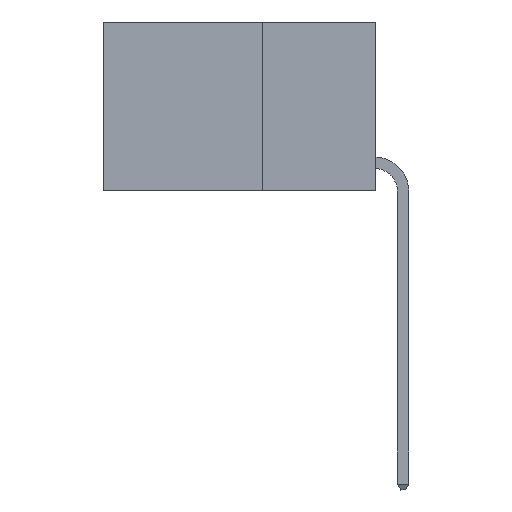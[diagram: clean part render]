
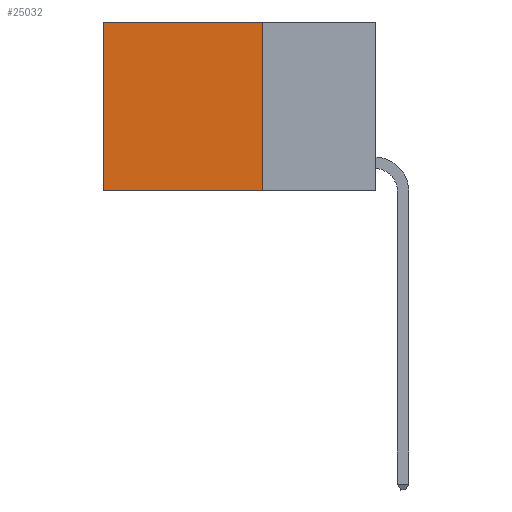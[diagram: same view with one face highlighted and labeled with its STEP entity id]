
A CAD part, left-side view. The second image highlights one B-rep face of the part: STEP entity #25032.
In plain terms, the highlighted planar face has unit normal (-1, 0, 0).
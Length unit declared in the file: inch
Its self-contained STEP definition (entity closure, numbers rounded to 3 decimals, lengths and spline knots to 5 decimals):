
#619 = CARTESIAN_POINT ( 'NONE',  ( 0.2625, 0.25, -0.37 ) ) ;
#737 = CARTESIAN_POINT ( 'NONE',  ( 0.2625, 0.25, 0. ) ) ;
#988 = DIRECTION ( 'NONE',  ( 1., 0., 0. ) ) ;
#2567 = VERTEX_POINT ( 'NONE', #619 ) ;
#2684 = EDGE_CURVE ( 'NONE', #2567, #5349, #3998, .T. ) ;
#3791 = PLANE ( 'NONE',  #26484 ) ;
#3998 = LINE ( 'NONE', #17075, #23084 ) ;
#4305 = VECTOR ( 'NONE', #7514, 39.37008 ) ;
#5349 = VERTEX_POINT ( 'NONE', #15169 ) ;
#5687 = VERTEX_POINT ( 'NONE', #18814 ) ;
#7514 = DIRECTION ( 'NONE',  ( 0., 0., -1. ) ) ;
#8128 = CARTESIAN_POINT ( 'NONE',  ( 0.2625, 0.25, 0. ) ) ;
#8396 = VERTEX_POINT ( 'NONE', #26364 ) ;
#9155 = ORIENTED_EDGE ( 'NONE', *, *, #14812, .T. ) ;
#10026 = LINE ( 'NONE', #8128, #20273 ) ;
#11539 = ORIENTED_EDGE ( 'NONE', *, *, #2684, .F. ) ;
#13070 = EDGE_LOOP ( 'NONE', ( #9155, #11539, #15220, #28313 ) ) ;
#14812 = EDGE_CURVE ( 'NONE', #5687, #5349, #15633, .T. ) ;
#15169 = CARTESIAN_POINT ( 'NONE',  ( 0.2625, 0.6, -0.37 ) ) ;
#15220 = ORIENTED_EDGE ( 'NONE', *, *, #20868, .F. ) ;
#15633 = LINE ( 'NONE', #24449, #18822 ) ;
#17075 = CARTESIAN_POINT ( 'NONE',  ( 0.2625, 0.25, -0.37 ) ) ;
#18814 = CARTESIAN_POINT ( 'NONE',  ( 0.2625, 0.6, 0. ) ) ;
#18822 = VECTOR ( 'NONE', #22367, 39.37008 ) ;
#20273 = VECTOR ( 'NONE', #21342, 39.37008 ) ;
#20622 = EDGE_CURVE ( 'NONE', #8396, #5687, #10026, .T. ) ;
#20868 = EDGE_CURVE ( 'NONE', #8396, #2567, #25427, .T. ) ;
#21268 = DIRECTION ( 'NONE',  ( 0., 0., -1. ) ) ;
#21342 = DIRECTION ( 'NONE',  ( 0., 1., 0. ) ) ;
#21624 = DIRECTION ( 'NONE',  ( 0., 1., 0. ) ) ;
#22367 = DIRECTION ( 'NONE',  ( 0., 0., -1. ) ) ;
#23084 = VECTOR ( 'NONE', #21624, 39.37008 ) ;
#23598 = CARTESIAN_POINT ( 'NONE',  ( 0.2625, 0.25, 0. ) ) ;
#24449 = CARTESIAN_POINT ( 'NONE',  ( 0.2625, 0.6, 0. ) ) ;
#25032 = ADVANCED_FACE ( 'NONE', ( #28303 ), #3791, .F. ) ;
#25427 = LINE ( 'NONE', #737, #4305 ) ;
#26364 = CARTESIAN_POINT ( 'NONE',  ( 0.2625, 0.25, 0. ) ) ;
#26484 = AXIS2_PLACEMENT_3D ( 'NONE', #23598, #988, #21268 ) ;
#28303 = FACE_OUTER_BOUND ( 'NONE', #13070, .T. ) ;
#28313 = ORIENTED_EDGE ( 'NONE', *, *, #20622, .T. ) ;
